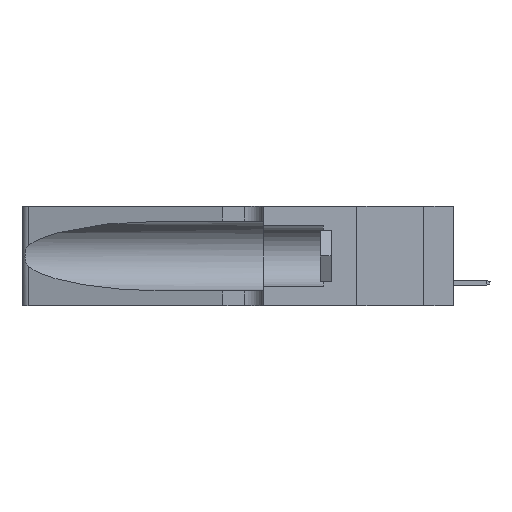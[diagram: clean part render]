
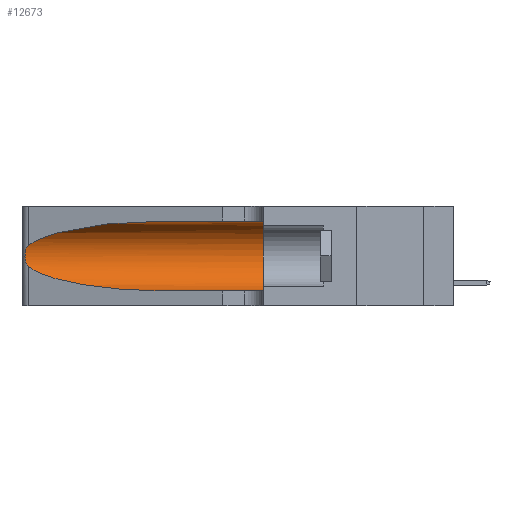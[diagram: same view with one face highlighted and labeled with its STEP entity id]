
A CAD part, left-side view. The second image highlights one B-rep face of the part: STEP entity #12673.
In plain terms, the highlighted cylindrical face has radius 3.308 mm (diameter 6.617 mm), a partial arc.
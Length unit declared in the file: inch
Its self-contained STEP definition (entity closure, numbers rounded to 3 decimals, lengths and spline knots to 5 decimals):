
#519 = CARTESIAN_POINT ( 'NONE',  ( 0.25639, 1.23186, 0.15144 ) ) ;
#560 = DIRECTION ( 'NONE',  ( 0., -1., 0. ) ) ;
#967 = CARTESIAN_POINT ( 'NONE',  ( 0.1305, 0.35, 0.31525 ) ) ;
#1455 = AXIS2_PLACEMENT_3D ( 'NONE', #46589, #7836, #34445 ) ;
#1946 = VERTEX_POINT ( 'NONE', #40631 ) ;
#2137 = ORIENTED_EDGE ( 'NONE', *, *, #12265, .T. ) ;
#3613 = CARTESIAN_POINT ( 'NONE',  ( 0.1305, 0.72297, 0.31525 ) ) ;
#3960 = EDGE_CURVE ( 'NONE', #39652, #16965, #6503, .T. ) ;
#4335 = EDGE_CURVE ( 'NONE', #7814, #14436, #35479, .T. ) ;
#4626 = DIRECTION ( 'NONE',  ( 0., 1., 0. ) ) ;
#5560 = CARTESIAN_POINT ( 'NONE',  ( 0.18966, 0.96281, 0.05475 ) ) ;
#5838 = CARTESIAN_POINT ( 'NONE',  ( 0.1305, 0.35, 0.05475 ) ) ;
#6503 = CIRCLE ( 'NONE', #19390, 0.13025 ) ;
#7510 = ORIENTED_EDGE ( 'NONE', *, *, #32607, .T. ) ;
#7814 = VERTEX_POINT ( 'NONE', #30849 ) ;
#7836 = DIRECTION ( 'NONE',  ( 0., -1., 0. ) ) ;
#8359 = CARTESIAN_POINT ( 'NONE',  ( 0.2373, 1.15595, 0.08982 ) ) ;
#11415 = LINE ( 'NONE', #23077, #32934 ) ;
#11638 = CARTESIAN_POINT ( 'NONE',  ( 0.26017, 1.23833, 0.17102 ) ) ;
#12265 = EDGE_CURVE ( 'NONE', #1946, #16965, #11415, .T. ) ;
#12649 = CARTESIAN_POINT ( 'NONE',  ( 0.25487, 1.22718, 0.14631 ) ) ;
#12673 = ADVANCED_FACE ( 'NONE', ( #18954 ), #27061, .F. ) ;
#12870 = CARTESIAN_POINT ( 'NONE',  ( 0.18966, 0.96281, 0.31525 ) ) ;
#14436 = VERTEX_POINT ( 'NONE', #46301 ) ;
#15927 = CARTESIAN_POINT ( 'NONE',  ( 0.25555, 1.22993, 0.14849 ) ) ;
#16226 = CARTESIAN_POINT ( 'NONE',  ( 0.1305, 1.61858, 0.31525 ) ) ;
#16965 = VERTEX_POINT ( 'NONE', #5838 ) ;
#18954 = FACE_OUTER_BOUND ( 'NONE', #24519, .T. ) ;
#19390 = AXIS2_PLACEMENT_3D ( 'NONE', #40062, #4626, #31457 ) ;
#20023 = LINE ( 'NONE', #16226, #38976 ) ;
#20722 = CARTESIAN_POINT ( 'NONE',  ( 0.1305, 0.72297, 0.31525 ) ) ;
#21458 = CARTESIAN_POINT ( 'NONE',  ( 0.2373, 1.15595, 0.28018 ) ) ;
#22801 = CARTESIAN_POINT ( 'NONE',  ( 0.25487, 1.22718, 0.22369 ) ) ;
#23077 = CARTESIAN_POINT ( 'NONE',  ( 0.1305, 1.61858, 0.05475 ) ) ;
#24519 = EDGE_LOOP ( 'NONE', ( #7510, #27150, #25104, #2137, #36214, #38972 ) ) ;
#25104 = ORIENTED_EDGE ( 'NONE', *, *, #39164, .T. ) ;
#26100 = CARTESIAN_POINT ( 'NONE',  ( 0.25787, 1.23484, 0.2124 ) ) ;
#26832 = CARTESIAN_POINT ( 'NONE',  ( 0.25555, 1.22994, 0.2215 ) ) ;
#27061 = CYLINDRICAL_SURFACE ( 'NONE', #1455, 0.13025 ) ;
#27150 = ORIENTED_EDGE ( 'NONE', *, *, #4335, .T. ) ;
#30849 = CARTESIAN_POINT ( 'NONE',  ( 0.25487, 1.22718, 0.22369 ) ) ;
#31457 = DIRECTION ( 'NONE',  ( 0., 0., 1. ) ) ;
#31699 = DIRECTION ( 'NONE',  ( 0., -1., 0. ) ) ;
#32607 = EDGE_CURVE ( 'NONE', #49428, #7814, #41228, .T. ) ;
#32642 = CARTESIAN_POINT ( 'NONE',  ( 0.25487, 1.22718, 0.22369 ) ) ;
#32934 = VECTOR ( 'NONE', #560, 39.37008 ) ;
#34445 = DIRECTION ( 'NONE',  ( 0., 0., -1. ) ) ;
#34695 = CARTESIAN_POINT ( 'NONE',  ( 0.26075, 1.23896, 0.19203 ) ) ;
#35206 = CARTESIAN_POINT ( 'NONE',  ( 0.25856, 1.23593, 0.16098 ) ) ;
#35479 = B_SPLINE_CURVE_WITH_KNOTS ( 'NONE', 3,
 ( #22801, #26832, #45371, #26100, #42319, #46373, #34695, #41579, #11638, #35206, #43588, #519, #15927, #42807 ),
 .UNSPECIFIED., .F., .F.,
 ( 4, 2, 2, 2, 2, 2, 4 ),
 ( 0., 0.00027, 0.00053, 0.00107, 0.0016, 0.00187, 0.00214 ),
 .UNSPECIFIED. ) ;
#36214 = ORIENTED_EDGE ( 'NONE', *, *, #3960, .F. ) ;
#36260 = EDGE_CURVE ( 'NONE', #49428, #39652, #20023, .T. ) ;
#38972 = ORIENTED_EDGE ( 'NONE', *, *, #36260, .F. ) ;
#38976 = VECTOR ( 'NONE', #31699, 39.37008 ) ;
#39164 = EDGE_CURVE ( 'NONE', #14436, #1946, #46410, .T. ) ;
#39652 = VERTEX_POINT ( 'NONE', #967 ) ;
#40062 = CARTESIAN_POINT ( 'NONE',  ( 0.1305, 0.35, 0.185 ) ) ;
#40631 = CARTESIAN_POINT ( 'NONE',  ( 0.1305, 0.72297, 0.05475 ) ) ;
#41228 =( BOUNDED_CURVE ( )  B_SPLINE_CURVE ( 3, ( #20722, #12870, #21458, #32642 ),
 .UNSPECIFIED., .F., .T. ) 
 B_SPLINE_CURVE_WITH_KNOTS ( ( 4, 4 ),
 ( 1.5708, 2.84003 ),
 .UNSPECIFIED. ) 
 CURVE ( )  GEOMETRIC_REPRESENTATION_ITEM ( )  RATIONAL_B_SPLINE_CURVE ( ( 1., 0.87, 0.87, 1. ) ) 
 REPRESENTATION_ITEM ( '' )  );
#41579 = CARTESIAN_POINT ( 'NONE',  ( 0.26075, 1.23896, 0.178 ) ) ;
#42319 = CARTESIAN_POINT ( 'NONE',  ( 0.25854, 1.2359, 0.20912 ) ) ;
#42807 = CARTESIAN_POINT ( 'NONE',  ( 0.25487, 1.22718, 0.14631 ) ) ;
#43588 = CARTESIAN_POINT ( 'NONE',  ( 0.25789, 1.23486, 0.15765 ) ) ;
#45371 = CARTESIAN_POINT ( 'NONE',  ( 0.25639, 1.23184, 0.21858 ) ) ;
#46301 = CARTESIAN_POINT ( 'NONE',  ( 0.25487, 1.22718, 0.14631 ) ) ;
#46373 = CARTESIAN_POINT ( 'NONE',  ( 0.26018, 1.23835, 0.19895 ) ) ;
#46410 =( BOUNDED_CURVE ( )  B_SPLINE_CURVE ( 3, ( #12649, #8359, #5560, #47613 ),
 .UNSPECIFIED., .F., .T. ) 
 B_SPLINE_CURVE_WITH_KNOTS ( ( 4, 4 ),
 ( 3.44316, 4.71239 ),
 .UNSPECIFIED. ) 
 CURVE ( )  GEOMETRIC_REPRESENTATION_ITEM ( )  RATIONAL_B_SPLINE_CURVE ( ( 1., 0.87, 0.87, 1. ) ) 
 REPRESENTATION_ITEM ( '' )  );
#46589 = CARTESIAN_POINT ( 'NONE',  ( 0.1305, 1.61858, 0.185 ) ) ;
#47613 = CARTESIAN_POINT ( 'NONE',  ( 0.1305, 0.72297, 0.05475 ) ) ;
#49428 = VERTEX_POINT ( 'NONE', #3613 ) ;
